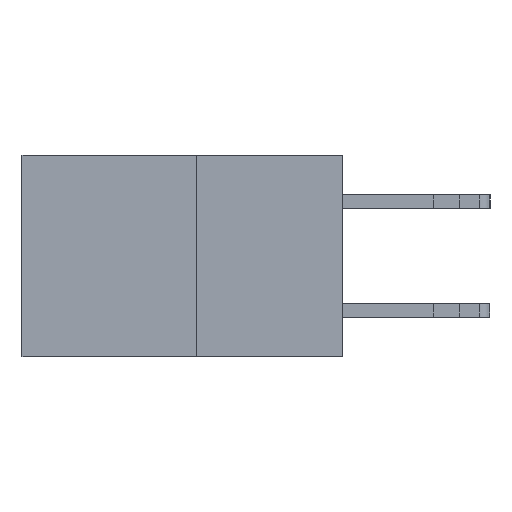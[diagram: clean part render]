
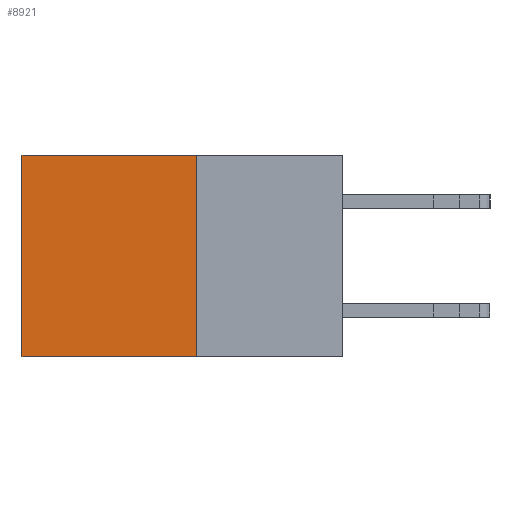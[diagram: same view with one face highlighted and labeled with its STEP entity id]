
A CAD part, left-side view. The second image highlights one B-rep face of the part: STEP entity #8921.
In plain terms, the highlighted planar face has unit normal (-1, 0, 0).
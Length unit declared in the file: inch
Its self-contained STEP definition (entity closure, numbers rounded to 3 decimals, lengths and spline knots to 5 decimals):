
#1675 = CARTESIAN_POINT ( 'NONE',  ( 0.277, 0.27, -0.37 ) ) ;
#3163 = VECTOR ( 'NONE', #6545, 39.37008 ) ;
#3495 = EDGE_CURVE ( 'NONE', #19668, #17775, #13299, .T. ) ;
#4555 = LINE ( 'NONE', #22375, #20739 ) ;
#4745 = ORIENTED_EDGE ( 'NONE', *, *, #5938, .T. ) ;
#5938 = EDGE_CURVE ( 'NONE', #8071, #19279, #18789, .T. ) ;
#5949 = FACE_OUTER_BOUND ( 'NONE', #9076, .T. ) ;
#6545 = DIRECTION ( 'NONE',  ( 0., 0., -1. ) ) ;
#6795 = PLANE ( 'NONE',  #14452 ) ;
#8071 = VERTEX_POINT ( 'NONE', #12750 ) ;
#8835 = DIRECTION ( 'NONE',  ( 0., 0., -1. ) ) ;
#8921 = ADVANCED_FACE ( 'NONE', ( #5949 ), #6795, .F. ) ;
#9076 = EDGE_LOOP ( 'NONE', ( #4745, #26288, #13304, #16402 ) ) ;
#10252 = CARTESIAN_POINT ( 'NONE',  ( 0.277, 0.27, -0.37 ) ) ;
#12274 = DIRECTION ( 'NONE',  ( 0., 1., 0. ) ) ;
#12750 = CARTESIAN_POINT ( 'NONE',  ( 0.277, 0.59, 0. ) ) ;
#13299 = LINE ( 'NONE', #18952, #3163 ) ;
#13304 = ORIENTED_EDGE ( 'NONE', *, *, #3495, .F. ) ;
#14452 = AXIS2_PLACEMENT_3D ( 'NONE', #14851, #20992, #8835 ) ;
#14851 = CARTESIAN_POINT ( 'NONE',  ( 0.277, 0.27, -0.37 ) ) ;
#14975 = EDGE_CURVE ( 'NONE', #17775, #19279, #15295, .T. ) ;
#15295 = LINE ( 'NONE', #10252, #20724 ) ;
#16402 = ORIENTED_EDGE ( 'NONE', *, *, #22663, .T. ) ;
#16538 = CARTESIAN_POINT ( 'NONE',  ( 0.277, 0.27, 0. ) ) ;
#17775 = VERTEX_POINT ( 'NONE', #1675 ) ;
#18789 = LINE ( 'NONE', #22419, #23543 ) ;
#18952 = CARTESIAN_POINT ( 'NONE',  ( 0.277, 0.27, -0.37 ) ) ;
#19279 = VERTEX_POINT ( 'NONE', #23672 ) ;
#19668 = VERTEX_POINT ( 'NONE', #16538 ) ;
#20724 = VECTOR ( 'NONE', #22392, 39.37008 ) ;
#20739 = VECTOR ( 'NONE', #12274, 39.37008 ) ;
#20992 = DIRECTION ( 'NONE',  ( 1., 0., 0. ) ) ;
#22375 = CARTESIAN_POINT ( 'NONE',  ( 0.277, 0.27, 0. ) ) ;
#22392 = DIRECTION ( 'NONE',  ( 0., 1., 0. ) ) ;
#22419 = CARTESIAN_POINT ( 'NONE',  ( 0.277, 0.59, -0.37 ) ) ;
#22663 = EDGE_CURVE ( 'NONE', #19668, #8071, #4555, .T. ) ;
#23543 = VECTOR ( 'NONE', #24474, 39.37008 ) ;
#23672 = CARTESIAN_POINT ( 'NONE',  ( 0.277, 0.59, -0.37 ) ) ;
#24474 = DIRECTION ( 'NONE',  ( 0., 0., -1. ) ) ;
#26288 = ORIENTED_EDGE ( 'NONE', *, *, #14975, .F. ) ;
